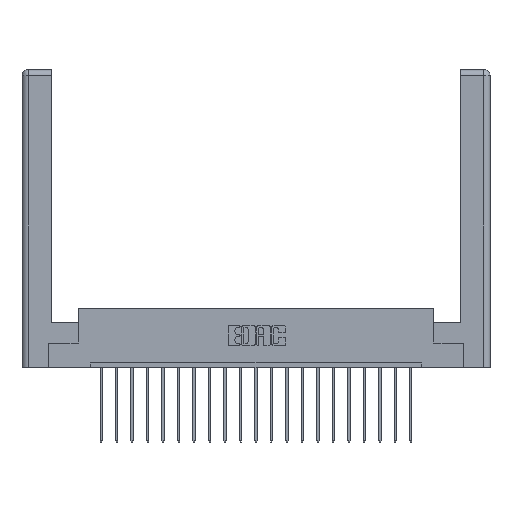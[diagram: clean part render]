
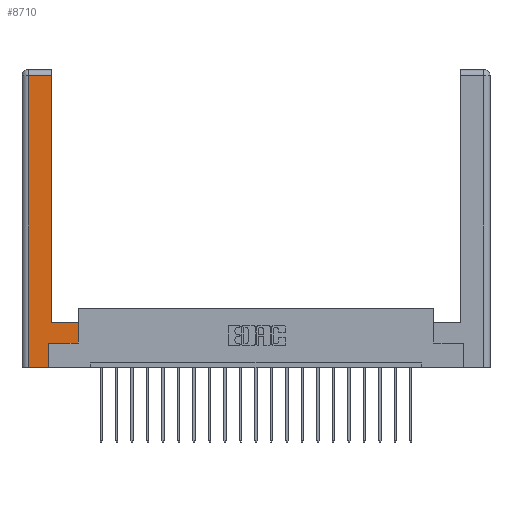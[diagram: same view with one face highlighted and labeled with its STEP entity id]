
A CAD part, top view. The second image highlights one B-rep face of the part: STEP entity #8710.
In plain terms, the highlighted planar face has unit normal (0, 0, 1).
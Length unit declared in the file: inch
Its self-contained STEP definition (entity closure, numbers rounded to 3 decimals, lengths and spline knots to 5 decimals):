
#45 = VECTOR ( 'NONE', #7234, 39.37008 ) ;
#396 = EDGE_CURVE ( 'NONE', #20523, #12606, #5425, .T. ) ;
#438 = CARTESIAN_POINT ( 'NONE',  ( 0.0615, 0., 0. ) ) ;
#644 = VECTOR ( 'NONE', #687, 39.37008 ) ;
#687 = DIRECTION ( 'NONE',  ( 0., 1., 0. ) ) ;
#831 = CARTESIAN_POINT ( 'NONE',  ( 0.265, 0.245, 0. ) ) ;
#924 = CARTESIAN_POINT ( 'NONE',  ( 0.565, 0.245, 0. ) ) ;
#1252 = CARTESIAN_POINT ( 'NONE',  ( 0.295, 0.45, 0. ) ) ;
#1257 = LINE ( 'NONE', #17653, #13105 ) ;
#1291 = DIRECTION ( 'NONE',  ( 0., 0., -1. ) ) ;
#1514 = LINE ( 'NONE', #1252, #9074 ) ;
#1541 = DIRECTION ( 'NONE',  ( -1., 0., 0. ) ) ;
#3000 = ORIENTED_EDGE ( 'NONE', *, *, #5213, .T. ) ;
#3255 = CARTESIAN_POINT ( 'NONE',  ( 0.295, 3., 0. ) ) ;
#3390 = VERTEX_POINT ( 'NONE', #11052 ) ;
#3401 = DIRECTION ( 'NONE',  ( 0., 1., 0. ) ) ;
#3460 = EDGE_CURVE ( 'NONE', #7716, #3390, #1514, .T. ) ;
#3471 = VERTEX_POINT ( 'NONE', #17740 ) ;
#3751 = CARTESIAN_POINT ( 'NONE',  ( 0.565, 0.45, 0. ) ) ;
#3795 = EDGE_CURVE ( 'NONE', #3390, #3471, #6774, .T. ) ;
#3922 = VECTOR ( 'NONE', #20917, 39.37008 ) ;
#4355 = CARTESIAN_POINT ( 'NONE',  ( 0.0615, 2.94, 0. ) ) ;
#5167 = VERTEX_POINT ( 'NONE', #12343 ) ;
#5213 = EDGE_CURVE ( 'NONE', #9400, #20523, #19291, .T. ) ;
#5425 = LINE ( 'NONE', #19493, #3922 ) ;
#6067 = EDGE_CURVE ( 'NONE', #5167, #6326, #19494, .T. ) ;
#6326 = VERTEX_POINT ( 'NONE', #15162 ) ;
#6774 = LINE ( 'NONE', #3255, #7279 ) ;
#7007 = VECTOR ( 'NONE', #14044, 39.37008 ) ;
#7234 = DIRECTION ( 'NONE',  ( 0., -1., 0. ) ) ;
#7279 = VECTOR ( 'NONE', #3401, 39.37008 ) ;
#7286 = ORIENTED_EDGE ( 'NONE', *, *, #3460, .T. ) ;
#7353 = ORIENTED_EDGE ( 'NONE', *, *, #6067, .T. ) ;
#7571 = VECTOR ( 'NONE', #12250, 39.37008 ) ;
#7712 = PLANE ( 'NONE',  #18364 ) ;
#7716 = VERTEX_POINT ( 'NONE', #3751 ) ;
#7940 = DIRECTION ( 'NONE',  ( 0., 1., 0. ) ) ;
#7989 = EDGE_CURVE ( 'NONE', #12606, #5167, #18625, .T. ) ;
#8710 = ADVANCED_FACE ( 'NONE', ( #10710 ), #7712, .F. ) ;
#9007 = CARTESIAN_POINT ( 'NONE',  ( 0.0615, 0., 0. ) ) ;
#9074 = VECTOR ( 'NONE', #1541, 39.37008 ) ;
#9336 = CARTESIAN_POINT ( 'NONE',  ( 0., 0., 0. ) ) ;
#9400 = VERTEX_POINT ( 'NONE', #18856 ) ;
#10710 = FACE_OUTER_BOUND ( 'NONE', #19278, .T. ) ;
#11052 = CARTESIAN_POINT ( 'NONE',  ( 0.295, 0.45, 0. ) ) ;
#11197 = CARTESIAN_POINT ( 'NONE',  ( 0.265, 0., 0. ) ) ;
#11337 = ORIENTED_EDGE ( 'NONE', *, *, #12393, .T. ) ;
#12250 = DIRECTION ( 'NONE',  ( 1., 0., 0. ) ) ;
#12343 = CARTESIAN_POINT ( 'NONE',  ( 0.265, 0.245, 0. ) ) ;
#12393 = EDGE_CURVE ( 'NONE', #3471, #9400, #16663, .T. ) ;
#12491 = ORIENTED_EDGE ( 'NONE', *, *, #7989, .T. ) ;
#12606 = VERTEX_POINT ( 'NONE', #11197 ) ;
#13105 = VECTOR ( 'NONE', #7940, 39.37008 ) ;
#14044 = DIRECTION ( 'NONE',  ( -1., 0., 0. ) ) ;
#15162 = CARTESIAN_POINT ( 'NONE',  ( 0.565, 0.245, 0. ) ) ;
#16663 = LINE ( 'NONE', #4355, #7007 ) ;
#17653 = CARTESIAN_POINT ( 'NONE',  ( 0.565, 0.45, 0. ) ) ;
#17740 = CARTESIAN_POINT ( 'NONE',  ( 0.295, 2.94, 0. ) ) ;
#18364 = AXIS2_PLACEMENT_3D ( 'NONE', #9336, #1291, #20674 ) ;
#18625 = LINE ( 'NONE', #831, #644 ) ;
#18856 = CARTESIAN_POINT ( 'NONE',  ( 0.0615, 2.94, 0. ) ) ;
#19278 = EDGE_LOOP ( 'NONE', ( #20537, #11337, #3000, #20286, #12491, #7353, #20069, #7286 ) ) ;
#19291 = LINE ( 'NONE', #9007, #45 ) ;
#19493 = CARTESIAN_POINT ( 'NONE',  ( 0.265, 0., 0. ) ) ;
#19494 = LINE ( 'NONE', #924, #7571 ) ;
#20069 = ORIENTED_EDGE ( 'NONE', *, *, #20293, .T. ) ;
#20286 = ORIENTED_EDGE ( 'NONE', *, *, #396, .T. ) ;
#20293 = EDGE_CURVE ( 'NONE', #6326, #7716, #1257, .T. ) ;
#20523 = VERTEX_POINT ( 'NONE', #438 ) ;
#20537 = ORIENTED_EDGE ( 'NONE', *, *, #3795, .T. ) ;
#20674 = DIRECTION ( 'NONE',  ( -1., 0., 0. ) ) ;
#20917 = DIRECTION ( 'NONE',  ( 1., 0., 0. ) ) ;
